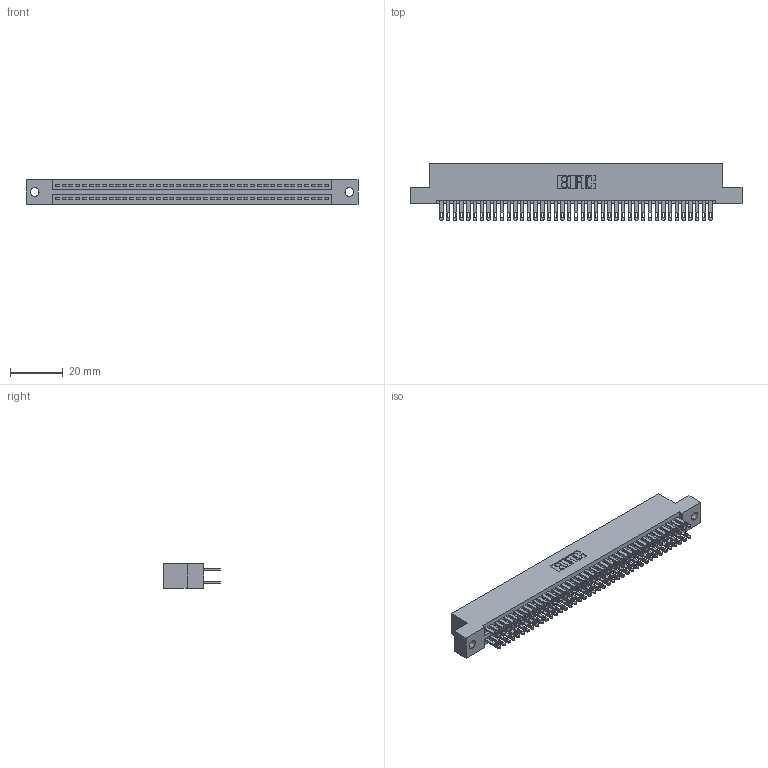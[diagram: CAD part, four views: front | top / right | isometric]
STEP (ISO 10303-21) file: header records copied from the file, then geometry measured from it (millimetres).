
FILE_DESCRIPTION (( 'STEP AP203' ), '1' );
FILE_NAME ('345-082-500-202.STEP', '2019-10-31T21:21:45', ( '' ), ( '' ), 'SwSTEP 2.0', 'SolidWorks 2016', '' );
FILE_SCHEMA (( 'CONFIG_CONTROL_DESIGN' ));
Length unit declared in the file: inch
Products named in the file (3): 345-082-500-202; 345-292-001_345-293-100; 345 Part_Flush Mounting Lugs - 0.128 Dia
Assembly tree (83 placements, depth 2):
  345-082-500-202
    345 Part_Flush Mounting Lugs - 0.128 Dia
    345-292-001_345-293-100  x82
Bounding box: 125.35 x 21.51 x 9.4 mm (x, y, z)
Volume: 12381.1 mm3; surface area: 18845.7 mm2
Topology: 83 solids, 83 shells, 3898 faces, 11903 edges, 7934 vertices
Faces by surface type: plane 2294, cylinder 1604
Entity records: 32237 total; most frequent: CARTESIAN_POINT 5404, ORIENTED_EDGE 5338, DIRECTION 4769, EDGE_CURVE 2669, VECTOR 2369, LINE 2369, VERTEX_POINT 1778, AXIS2_PLACEMENT_3D 1200
